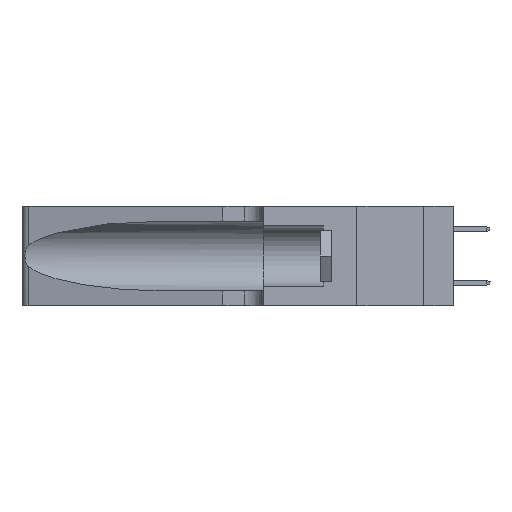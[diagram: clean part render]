
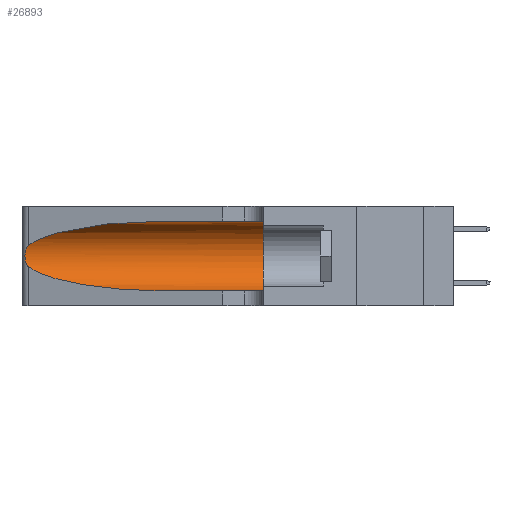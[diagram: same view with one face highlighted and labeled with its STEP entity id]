
A CAD part, left-side view. The second image highlights one B-rep face of the part: STEP entity #26893.
In plain terms, the highlighted cylindrical face has radius 3.308 mm (diameter 6.617 mm), a partial arc.
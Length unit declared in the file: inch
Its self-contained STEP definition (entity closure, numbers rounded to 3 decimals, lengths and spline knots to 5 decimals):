
#434 = DIRECTION ( 'NONE',  ( 0., 0., 1. ) ) ;
#806 = VERTEX_POINT ( 'NONE', #13142 ) ;
#1201 = ORIENTED_EDGE ( 'NONE', *, *, #18443, .T. ) ;
#1347 = CARTESIAN_POINT ( 'NONE',  ( 0.25555, 1.22994, 0.2215 ) ) ;
#1394 = AXIS2_PLACEMENT_3D ( 'NONE', #21277, #17729, #26036 ) ;
#2277 = CARTESIAN_POINT ( 'NONE',  ( 0.25487, 1.22718, 0.22369 ) ) ;
#2734 = CARTESIAN_POINT ( 'NONE',  ( 0.2373, 1.15595, 0.28018 ) ) ;
#3205 = EDGE_CURVE ( 'NONE', #7281, #12749, #6492, .T. ) ;
#3669 = CARTESIAN_POINT ( 'NONE',  ( 0.26018, 1.23835, 0.19895 ) ) ;
#4061 = CARTESIAN_POINT ( 'NONE',  ( 0.2373, 1.15595, 0.08982 ) ) ;
#4780 = CARTESIAN_POINT ( 'NONE',  ( 0.1305, 0.35, 0.31525 ) ) ;
#5121 = ORIENTED_EDGE ( 'NONE', *, *, #3205, .F. ) ;
#5451 = CARTESIAN_POINT ( 'NONE',  ( 0.25787, 1.23484, 0.2124 ) ) ;
#5828 = VECTOR ( 'NONE', #21142, 39.37008 ) ;
#6450 = CARTESIAN_POINT ( 'NONE',  ( 0.1305, 0.35, 0.185 ) ) ;
#6492 = LINE ( 'NONE', #25361, #5828 ) ;
#6623 = CARTESIAN_POINT ( 'NONE',  ( 0.1305, 0.72297, 0.31525 ) ) ;
#7072 = B_SPLINE_CURVE_WITH_KNOTS ( 'NONE', 3,
 ( #22429, #1347, #22153, #5451, #11534, #3669, #26519, #11955, #12079, #20387, #18354, #16580, #8550, #8017 ),
 .UNSPECIFIED., .F., .F.,
 ( 4, 2, 2, 2, 2, 2, 4 ),
 ( 0., 0.00027, 0.00053, 0.00107, 0.0016, 0.00187, 0.00214 ),
 .UNSPECIFIED. ) ;
#7140 = CYLINDRICAL_SURFACE ( 'NONE', #1394, 0.13025 ) ;
#7281 = VERTEX_POINT ( 'NONE', #6623 ) ;
#8017 = CARTESIAN_POINT ( 'NONE',  ( 0.25487, 1.22718, 0.14631 ) ) ;
#8407 = CARTESIAN_POINT ( 'NONE',  ( 0.1305, 0.72297, 0.05475 ) ) ;
#8550 = CARTESIAN_POINT ( 'NONE',  ( 0.25555, 1.22993, 0.14849 ) ) ;
#9724 = VERTEX_POINT ( 'NONE', #20255 ) ;
#10526 = ORIENTED_EDGE ( 'NONE', *, *, #24333, .T. ) ;
#11534 = CARTESIAN_POINT ( 'NONE',  ( 0.25854, 1.2359, 0.20912 ) ) ;
#11955 = CARTESIAN_POINT ( 'NONE',  ( 0.26075, 1.23896, 0.178 ) ) ;
#12068 = AXIS2_PLACEMENT_3D ( 'NONE', #6450, #21108, #434 ) ;
#12079 = CARTESIAN_POINT ( 'NONE',  ( 0.26017, 1.23833, 0.17102 ) ) ;
#12252 = VERTEX_POINT ( 'NONE', #14453 ) ;
#12749 = VERTEX_POINT ( 'NONE', #4780 ) ;
#13142 = CARTESIAN_POINT ( 'NONE',  ( 0.1305, 0.35, 0.05475 ) ) ;
#13181 = CARTESIAN_POINT ( 'NONE',  ( 0.18966, 0.96281, 0.31525 ) ) ;
#13854 = EDGE_LOOP ( 'NONE', ( #18398, #1201, #26811, #10526, #19009, #5121 ) ) ;
#14005 = LINE ( 'NONE', #18371, #24370 ) ;
#14380 = CARTESIAN_POINT ( 'NONE',  ( 0.18966, 0.96281, 0.05475 ) ) ;
#14453 = CARTESIAN_POINT ( 'NONE',  ( 0.1305, 0.72297, 0.05475 ) ) ;
#15571 = EDGE_CURVE ( 'NONE', #7281, #20858, #19248, .T. ) ;
#16284 = EDGE_CURVE ( 'NONE', #12749, #806, #24226, .T. ) ;
#16580 = CARTESIAN_POINT ( 'NONE',  ( 0.25639, 1.23186, 0.15144 ) ) ;
#17281 = CARTESIAN_POINT ( 'NONE',  ( 0.1305, 0.72297, 0.31525 ) ) ;
#17729 = DIRECTION ( 'NONE',  ( 0., -1., 0. ) ) ;
#17960 = DIRECTION ( 'NONE',  ( 0., -1., 0. ) ) ;
#18354 = CARTESIAN_POINT ( 'NONE',  ( 0.25789, 1.23486, 0.15765 ) ) ;
#18371 = CARTESIAN_POINT ( 'NONE',  ( 0.1305, 1.61858, 0.05475 ) ) ;
#18376 =( BOUNDED_CURVE ( )  B_SPLINE_CURVE ( 3, ( #22812, #4061, #14380, #8407 ),
 .UNSPECIFIED., .F., .T. ) 
 B_SPLINE_CURVE_WITH_KNOTS ( ( 4, 4 ),
 ( 3.44316, 4.71239 ),
 .UNSPECIFIED. ) 
 CURVE ( )  GEOMETRIC_REPRESENTATION_ITEM ( )  RATIONAL_B_SPLINE_CURVE ( ( 1., 0.87, 0.87, 1. ) ) 
 REPRESENTATION_ITEM ( '' )  );
#18398 = ORIENTED_EDGE ( 'NONE', *, *, #15571, .T. ) ;
#18443 = EDGE_CURVE ( 'NONE', #20858, #9724, #7072, .T. ) ;
#19009 = ORIENTED_EDGE ( 'NONE', *, *, #16284, .F. ) ;
#19248 =( BOUNDED_CURVE ( )  B_SPLINE_CURVE ( 3, ( #17281, #13181, #2734, #19714 ),
 .UNSPECIFIED., .F., .T. ) 
 B_SPLINE_CURVE_WITH_KNOTS ( ( 4, 4 ),
 ( 1.5708, 2.84003 ),
 .UNSPECIFIED. ) 
 CURVE ( )  GEOMETRIC_REPRESENTATION_ITEM ( )  RATIONAL_B_SPLINE_CURVE ( ( 1., 0.87, 0.87, 1. ) ) 
 REPRESENTATION_ITEM ( '' )  );
#19714 = CARTESIAN_POINT ( 'NONE',  ( 0.25487, 1.22718, 0.22369 ) ) ;
#20255 = CARTESIAN_POINT ( 'NONE',  ( 0.25487, 1.22718, 0.14631 ) ) ;
#20387 = CARTESIAN_POINT ( 'NONE',  ( 0.25856, 1.23593, 0.16098 ) ) ;
#20858 = VERTEX_POINT ( 'NONE', #2277 ) ;
#21108 = DIRECTION ( 'NONE',  ( 0., 1., 0. ) ) ;
#21142 = DIRECTION ( 'NONE',  ( 0., -1., 0. ) ) ;
#21277 = CARTESIAN_POINT ( 'NONE',  ( 0.1305, 1.61858, 0.185 ) ) ;
#22114 = EDGE_CURVE ( 'NONE', #9724, #12252, #18376, .T. ) ;
#22153 = CARTESIAN_POINT ( 'NONE',  ( 0.25639, 1.23184, 0.21858 ) ) ;
#22429 = CARTESIAN_POINT ( 'NONE',  ( 0.25487, 1.22718, 0.22369 ) ) ;
#22812 = CARTESIAN_POINT ( 'NONE',  ( 0.25487, 1.22718, 0.14631 ) ) ;
#24226 = CIRCLE ( 'NONE', #12068, 0.13025 ) ;
#24333 = EDGE_CURVE ( 'NONE', #12252, #806, #14005, .T. ) ;
#24370 = VECTOR ( 'NONE', #17960, 39.37008 ) ;
#25361 = CARTESIAN_POINT ( 'NONE',  ( 0.1305, 1.61858, 0.31525 ) ) ;
#25766 = FACE_OUTER_BOUND ( 'NONE', #13854, .T. ) ;
#26036 = DIRECTION ( 'NONE',  ( 0., 0., -1. ) ) ;
#26519 = CARTESIAN_POINT ( 'NONE',  ( 0.26075, 1.23896, 0.19203 ) ) ;
#26811 = ORIENTED_EDGE ( 'NONE', *, *, #22114, .T. ) ;
#26893 = ADVANCED_FACE ( 'NONE', ( #25766 ), #7140, .F. ) ;
